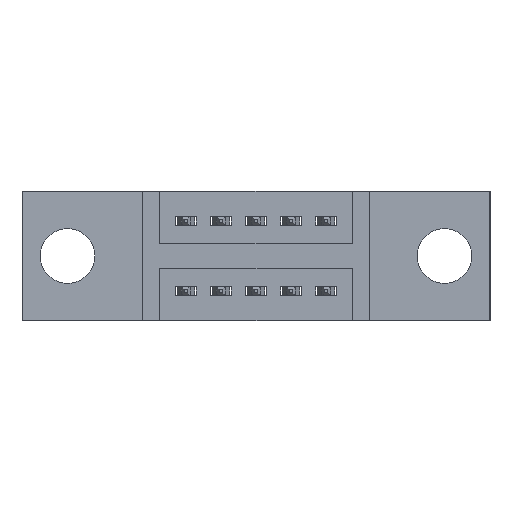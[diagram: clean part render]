
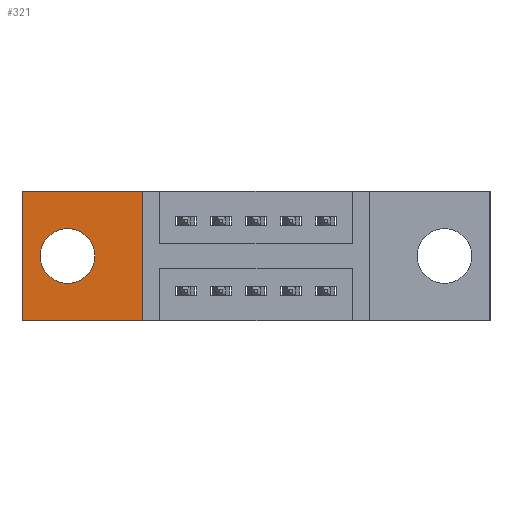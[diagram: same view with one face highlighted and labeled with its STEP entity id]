
A CAD part, front view. The second image highlights one B-rep face of the part: STEP entity #321.
In plain terms, the highlighted planar face has unit normal (0, -1, 0).
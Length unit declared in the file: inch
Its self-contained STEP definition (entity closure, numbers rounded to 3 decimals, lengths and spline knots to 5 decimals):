
#321 = ADVANCED_FACE ( 'NONE', ( #2379, #1920 ), #4856, .T. ) ;
#361 = CARTESIAN_POINT ( 'NONE',  ( 0.3425, 0.11, 0. ) ) ;
#407 = VERTEX_POINT ( 'NONE', #3336 ) ;
#542 = CARTESIAN_POINT ( 'NONE',  ( 0.13, 0.11, -0.107 ) ) ;
#882 = ORIENTED_EDGE ( 'NONE', *, *, #1337, .F. ) ;
#1315 = DIRECTION ( 'NONE',  ( -1., 0., 0. ) ) ;
#1337 = EDGE_CURVE ( 'NONE', #3226, #6195, #8170, .T. ) ;
#1453 = DIRECTION ( 'NONE',  ( 0., -1., 0. ) ) ;
#1787 = VECTOR ( 'NONE', #1315, 39.37008 ) ;
#1811 = DIRECTION ( 'NONE',  ( 0., 0., -1. ) ) ;
#1885 = DIRECTION ( 'NONE',  ( 0., -1., 0. ) ) ;
#1909 = DIRECTION ( 'NONE',  ( 0., -1., 0. ) ) ;
#1911 = CIRCLE ( 'NONE', #2985, 0.078 ) ;
#1920 = FACE_OUTER_BOUND ( 'NONE', #6561, .T. ) ;
#2268 = VERTEX_POINT ( 'NONE', #3035 ) ;
#2349 = DIRECTION ( 'NONE',  ( 1., 0., 0. ) ) ;
#2379 = FACE_BOUND ( 'NONE', #8118, .T. ) ;
#2985 = AXIS2_PLACEMENT_3D ( 'NONE', #8368, #1453, #4486 ) ;
#3035 = CARTESIAN_POINT ( 'NONE',  ( 0., 0.11, -0.37 ) ) ;
#3226 = VERTEX_POINT ( 'NONE', #542 ) ;
#3336 = CARTESIAN_POINT ( 'NONE',  ( 0.3425, 0.11, 0. ) ) ;
#3452 = DIRECTION ( 'NONE',  ( 0., 0., -1. ) ) ;
#3732 = DIRECTION ( 'NONE',  ( 0., 0., 1. ) ) ;
#3744 = AXIS2_PLACEMENT_3D ( 'NONE', #5220, #1885, #3452 ) ;
#3747 = AXIS2_PLACEMENT_3D ( 'NONE', #8159, #1909, #1811 ) ;
#4415 = CARTESIAN_POINT ( 'NONE',  ( 0., 0.11, 0. ) ) ;
#4486 = DIRECTION ( 'NONE',  ( 0., 0., -1. ) ) ;
#4652 = ORIENTED_EDGE ( 'NONE', *, *, #8793, .T. ) ;
#4745 = ORIENTED_EDGE ( 'NONE', *, *, #5789, .T. ) ;
#4765 = EDGE_CURVE ( 'NONE', #8207, #2268, #8924, .T. ) ;
#4856 = PLANE ( 'NONE',  #3744 ) ;
#4992 = LINE ( 'NONE', #361, #7293 ) ;
#5042 = EDGE_CURVE ( 'NONE', #2268, #9032, #9022, .T. ) ;
#5220 = CARTESIAN_POINT ( 'NONE',  ( 0., 0.11, -0.37 ) ) ;
#5611 = CARTESIAN_POINT ( 'NONE',  ( 0., 0.11, 0. ) ) ;
#5789 = EDGE_CURVE ( 'NONE', #407, #8207, #7817, .T. ) ;
#6089 = CARTESIAN_POINT ( 'NONE',  ( 0.13, 0.11, -0.263 ) ) ;
#6168 = EDGE_CURVE ( 'NONE', #6195, #3226, #1911, .T. ) ;
#6195 = VERTEX_POINT ( 'NONE', #6089 ) ;
#6240 = DIRECTION ( 'NONE',  ( 0., 0., -1. ) ) ;
#6317 = CARTESIAN_POINT ( 'NONE',  ( 0., 0.11, 0. ) ) ;
#6561 = EDGE_LOOP ( 'NONE', ( #8364, #7639, #4652, #4745 ) ) ;
#7060 = VECTOR ( 'NONE', #6240, 39.37008 ) ;
#7158 = VECTOR ( 'NONE', #2349, 39.37008 ) ;
#7293 = VECTOR ( 'NONE', #3732, 39.37008 ) ;
#7639 = ORIENTED_EDGE ( 'NONE', *, *, #5042, .T. ) ;
#7817 = LINE ( 'NONE', #4415, #1787 ) ;
#8118 = EDGE_LOOP ( 'NONE', ( #882, #8880 ) ) ;
#8159 = CARTESIAN_POINT ( 'NONE',  ( 0.13, 0.11, -0.185 ) ) ;
#8170 = CIRCLE ( 'NONE', #3747, 0.078 ) ;
#8207 = VERTEX_POINT ( 'NONE', #6317 ) ;
#8218 = CARTESIAN_POINT ( 'NONE',  ( 0.3425, 0.11, -0.37 ) ) ;
#8364 = ORIENTED_EDGE ( 'NONE', *, *, #4765, .T. ) ;
#8368 = CARTESIAN_POINT ( 'NONE',  ( 0.13, 0.11, -0.185 ) ) ;
#8746 = CARTESIAN_POINT ( 'NONE',  ( 0., 0.11, -0.37 ) ) ;
#8793 = EDGE_CURVE ( 'NONE', #9032, #407, #4992, .T. ) ;
#8880 = ORIENTED_EDGE ( 'NONE', *, *, #6168, .F. ) ;
#8924 = LINE ( 'NONE', #5611, #7060 ) ;
#9022 = LINE ( 'NONE', #8746, #7158 ) ;
#9032 = VERTEX_POINT ( 'NONE', #8218 ) ;
